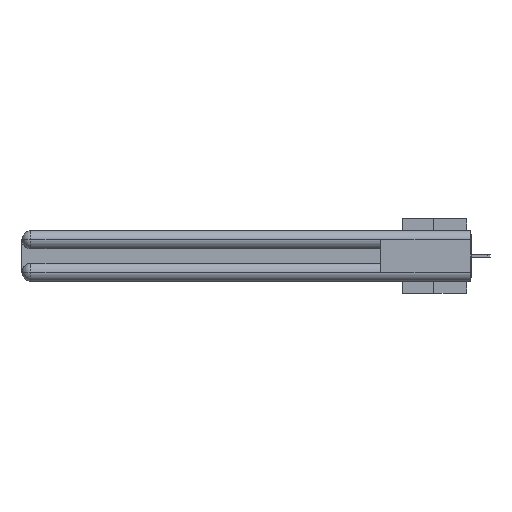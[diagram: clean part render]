
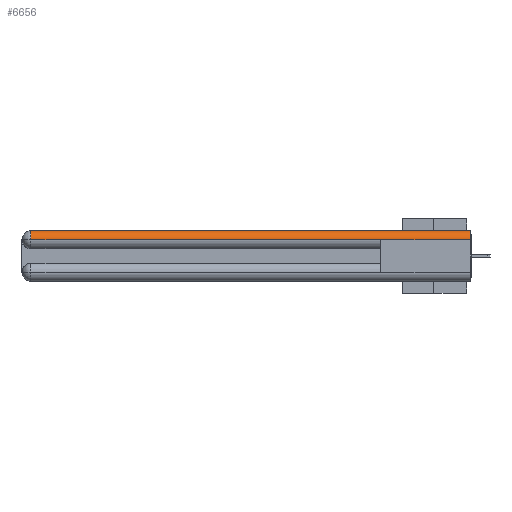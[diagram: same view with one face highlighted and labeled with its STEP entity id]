
A CAD part, left-side view. The second image highlights one B-rep face of the part: STEP entity #6656.
In plain terms, the highlighted cylindrical face has radius 1.562 mm (diameter 3.124 mm), a partial arc.
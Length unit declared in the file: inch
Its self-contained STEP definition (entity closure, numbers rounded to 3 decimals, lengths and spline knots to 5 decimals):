
#1250 = EDGE_CURVE ( 'NONE', #7678, #34260, #33552, .T. ) ;
#2592 = EDGE_CURVE ( 'NONE', #31283, #34260, #6221, .T. ) ;
#3205 = VECTOR ( 'NONE', #19188, 39.37008 ) ;
#4382 = ORIENTED_EDGE ( 'NONE', *, *, #18693, .F. ) ;
#6221 = LINE ( 'NONE', #40034, #24442 ) ;
#6428 = CARTESIAN_POINT ( 'NONE',  ( 0.0615, 0., -0.0615 ) ) ;
#6656 = ADVANCED_FACE ( 'NONE', ( #23856 ), #31332, .T. ) ;
#7678 = VERTEX_POINT ( 'NONE', #39255 ) ;
#9743 = DIRECTION ( 'NONE',  ( 1., 0., 0. ) ) ;
#10902 = CARTESIAN_POINT ( 'NONE',  ( 0.0615, 2.94, -0.0615 ) ) ;
#11130 = ORIENTED_EDGE ( 'NONE', *, *, #35855, .F. ) ;
#13896 = AXIS2_PLACEMENT_3D ( 'NONE', #10902, #33331, #14183 ) ;
#14183 = DIRECTION ( 'NONE',  ( 0., 0., 1. ) ) ;
#16136 = AXIS2_PLACEMENT_3D ( 'NONE', #6428, #29007, #9743 ) ;
#16557 = VECTOR ( 'NONE', #39099, 39.37008 ) ;
#17811 = CIRCLE ( 'NONE', #16136, 0.0615 ) ;
#18693 = EDGE_CURVE ( 'NONE', #37831, #38014, #21599, .T. ) ;
#19188 = DIRECTION ( 'NONE',  ( 0., -1., 0. ) ) ;
#21599 = LINE ( 'NONE', #28661, #3205 ) ;
#21849 = CARTESIAN_POINT ( 'NONE',  ( 0.0615, 0., 0. ) ) ;
#21857 = CARTESIAN_POINT ( 'NONE',  ( 0.0615, 0., -0.0615 ) ) ;
#23270 = CARTESIAN_POINT ( 'NONE',  ( 0., 3., -0.0615 ) ) ;
#23856 = FACE_OUTER_BOUND ( 'NONE', #37101, .T. ) ;
#24442 = VECTOR ( 'NONE', #27306, 39.37008 ) ;
#24595 = ORIENTED_EDGE ( 'NONE', *, *, #2592, .T. ) ;
#25049 = DIRECTION ( 'NONE',  ( 0., 0., 1. ) ) ;
#27306 = DIRECTION ( 'NONE',  ( 0., -1., 0. ) ) ;
#28661 = CARTESIAN_POINT ( 'NONE',  ( 0.0615, 0., 0. ) ) ;
#29007 = DIRECTION ( 'NONE',  ( 0., -1., 0. ) ) ;
#30346 = CARTESIAN_POINT ( 'NONE',  ( 0.0615, 2.94, 0. ) ) ;
#30969 = EDGE_CURVE ( 'NONE', #37831, #31283, #34169, .T. ) ;
#31283 = VERTEX_POINT ( 'NONE', #37091 ) ;
#31332 = CYLINDRICAL_SURFACE ( 'NONE', #33370, 0.0615 ) ;
#33155 = CARTESIAN_POINT ( 'NONE',  ( 0., 0.6, -0.0615 ) ) ;
#33331 = DIRECTION ( 'NONE',  ( 0., -1., 0. ) ) ;
#33370 = AXIS2_PLACEMENT_3D ( 'NONE', #21857, #37704, #25049 ) ;
#33552 = LINE ( 'NONE', #23270, #16557 ) ;
#34169 = CIRCLE ( 'NONE', #13896, 0.0615 ) ;
#34260 = VERTEX_POINT ( 'NONE', #33155 ) ;
#35855 = EDGE_CURVE ( 'NONE', #38014, #7678, #17811, .T. ) ;
#37091 = CARTESIAN_POINT ( 'NONE',  ( 0., 2.94, -0.0615 ) ) ;
#37101 = EDGE_LOOP ( 'NONE', ( #4382, #41598, #24595, #41427, #11130 ) ) ;
#37704 = DIRECTION ( 'NONE',  ( 0., 1., 0. ) ) ;
#37831 = VERTEX_POINT ( 'NONE', #30346 ) ;
#38014 = VERTEX_POINT ( 'NONE', #21849 ) ;
#39099 = DIRECTION ( 'NONE',  ( 0., 1., 0. ) ) ;
#39255 = CARTESIAN_POINT ( 'NONE',  ( 0., 0., -0.0615 ) ) ;
#40034 = CARTESIAN_POINT ( 'NONE',  ( 0., 3., -0.0615 ) ) ;
#41427 = ORIENTED_EDGE ( 'NONE', *, *, #1250, .F. ) ;
#41598 = ORIENTED_EDGE ( 'NONE', *, *, #30969, .T. ) ;
